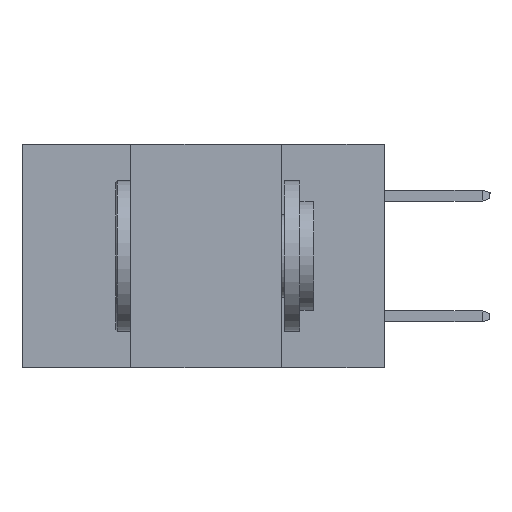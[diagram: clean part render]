
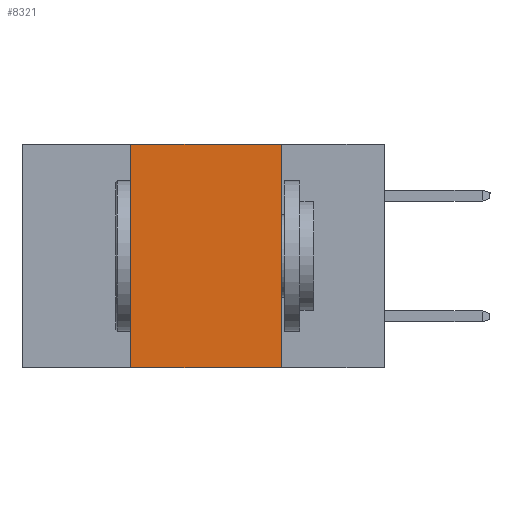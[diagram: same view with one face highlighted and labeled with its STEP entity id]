
A CAD part, left-side view. The second image highlights one B-rep face of the part: STEP entity #8321.
In plain terms, the highlighted planar face has unit normal (-1, 0, 0).
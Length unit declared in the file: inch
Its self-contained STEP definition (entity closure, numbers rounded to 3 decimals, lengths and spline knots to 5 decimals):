
#312 = DIRECTION ( 'NONE',  ( 0., 0., 1. ) ) ;
#1222 = VERTEX_POINT ( 'NONE', #3291 ) ;
#1280 = VECTOR ( 'NONE', #312, 39.37008 ) ;
#1592 = CARTESIAN_POINT ( 'NONE',  ( 0., 0.17, -0.37 ) ) ;
#1883 = VERTEX_POINT ( 'NONE', #12883 ) ;
#2501 = VECTOR ( 'NONE', #10728, 39.37008 ) ;
#2617 = PLANE ( 'NONE',  #15822 ) ;
#2805 = CARTESIAN_POINT ( 'NONE',  ( 0., 0.6, -0.37 ) ) ;
#3108 = LINE ( 'NONE', #17521, #8048 ) ;
#3291 = CARTESIAN_POINT ( 'NONE',  ( 0., 0.42, 0. ) ) ;
#3842 = VERTEX_POINT ( 'NONE', #18043 ) ;
#3905 = ORIENTED_EDGE ( 'NONE', *, *, #5594, .F. ) ;
#4402 = LINE ( 'NONE', #10160, #1280 ) ;
#5594 = EDGE_CURVE ( 'NONE', #3842, #12650, #17449, .T. ) ;
#5953 = EDGE_CURVE ( 'NONE', #1883, #1222, #4402, .T. ) ;
#6566 = EDGE_LOOP ( 'NONE', ( #3905, #7366, #10770, #11784 ) ) ;
#6847 = FACE_OUTER_BOUND ( 'NONE', #6566, .T. ) ;
#6930 = DIRECTION ( 'NONE',  ( 0., 0., -1. ) ) ;
#7366 = ORIENTED_EDGE ( 'NONE', *, *, #16853, .F. ) ;
#8048 = VECTOR ( 'NONE', #14865, 39.37008 ) ;
#8321 = ADVANCED_FACE ( 'NONE', ( #6847 ), #2617, .F. ) ;
#10160 = CARTESIAN_POINT ( 'NONE',  ( 0., 0.42, -0.37 ) ) ;
#10728 = DIRECTION ( 'NONE',  ( 0., 0., -1. ) ) ;
#10770 = ORIENTED_EDGE ( 'NONE', *, *, #5953, .F. ) ;
#11202 = DIRECTION ( 'NONE',  ( 0., -1., 0. ) ) ;
#11784 = ORIENTED_EDGE ( 'NONE', *, *, #15775, .T. ) ;
#12616 = CARTESIAN_POINT ( 'NONE',  ( 0., 0.6, 0. ) ) ;
#12650 = VERTEX_POINT ( 'NONE', #16935 ) ;
#12883 = CARTESIAN_POINT ( 'NONE',  ( 0., 0.42, -0.37 ) ) ;
#14099 = DIRECTION ( 'NONE',  ( 1., 0., 0. ) ) ;
#14865 = DIRECTION ( 'NONE',  ( 0., -1., 0. ) ) ;
#15704 = LINE ( 'NONE', #2805, #17050 ) ;
#15775 = EDGE_CURVE ( 'NONE', #1883, #12650, #15704, .T. ) ;
#15822 = AXIS2_PLACEMENT_3D ( 'NONE', #12616, #14099, #6930 ) ;
#16853 = EDGE_CURVE ( 'NONE', #1222, #3842, #3108, .T. ) ;
#16935 = CARTESIAN_POINT ( 'NONE',  ( 0., 0.17, -0.37 ) ) ;
#17050 = VECTOR ( 'NONE', #11202, 39.37008 ) ;
#17449 = LINE ( 'NONE', #1592, #2501 ) ;
#17521 = CARTESIAN_POINT ( 'NONE',  ( 0., 0.6, 0. ) ) ;
#18043 = CARTESIAN_POINT ( 'NONE',  ( 0., 0.17, 0. ) ) ;
